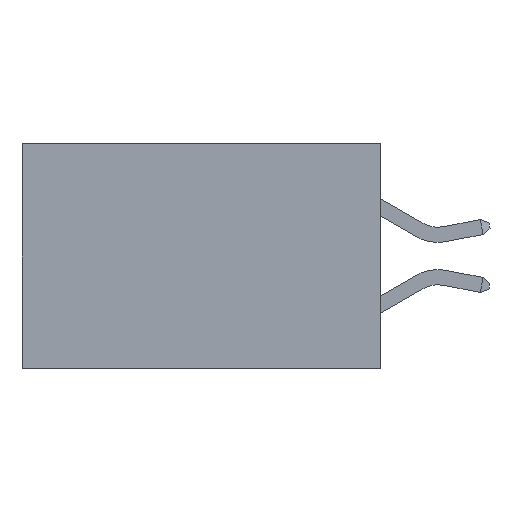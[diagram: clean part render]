
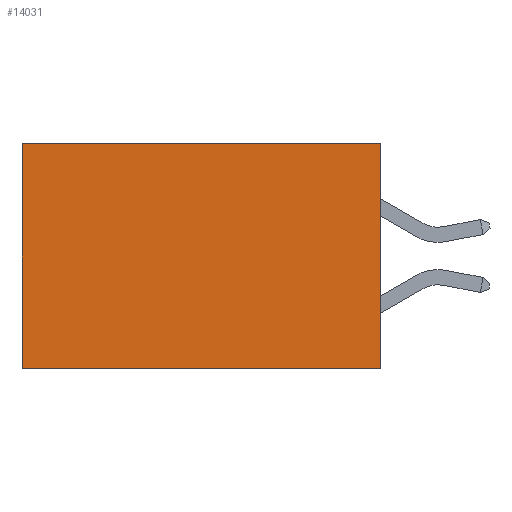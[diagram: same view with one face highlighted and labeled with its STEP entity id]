
A CAD part, left-side view. The second image highlights one B-rep face of the part: STEP entity #14031.
In plain terms, the highlighted planar face has unit normal (-1, 0, 0).
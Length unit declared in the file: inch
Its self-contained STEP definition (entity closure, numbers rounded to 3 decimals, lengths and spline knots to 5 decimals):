
#9 = EDGE_CURVE ( 'NONE', #14758, #8744, #9076, .T. ) ;
#296 = LINE ( 'NONE', #15651, #13128 ) ;
#1215 = AXIS2_PLACEMENT_3D ( 'NONE', #3953, #5200, #13872 ) ;
#1379 = VECTOR ( 'NONE', #11923, 39.37008 ) ;
#1619 = ORIENTED_EDGE ( 'NONE', *, *, #9367, .F. ) ;
#1762 = FACE_OUTER_BOUND ( 'NONE', #6398, .T. ) ;
#2040 = DIRECTION ( 'NONE',  ( 0., 1., 0. ) ) ;
#2311 = EDGE_CURVE ( 'NONE', #11370, #11696, #8771, .T. ) ;
#2517 = DIRECTION ( 'NONE',  ( 0., 0., -1. ) ) ;
#2707 = CARTESIAN_POINT ( 'NONE',  ( 0.277, 0., -0.37 ) ) ;
#3953 = CARTESIAN_POINT ( 'NONE',  ( 0.277, 0., -0.37 ) ) ;
#4618 = ORIENTED_EDGE ( 'NONE', *, *, #2311, .F. ) ;
#5199 = DIRECTION ( 'NONE',  ( 0., 1., 0. ) ) ;
#5200 = DIRECTION ( 'NONE',  ( 1., 0., 0. ) ) ;
#5404 = VECTOR ( 'NONE', #5199, 39.37008 ) ;
#6195 = EDGE_CURVE ( 'NONE', #11370, #14758, #296, .T. ) ;
#6398 = EDGE_LOOP ( 'NONE', ( #13866, #1619, #4618, #14774 ) ) ;
#6412 = PLANE ( 'NONE',  #1215 ) ;
#7197 = CARTESIAN_POINT ( 'NONE',  ( 0.277, 0., -0.37 ) ) ;
#8684 = LINE ( 'NONE', #2707, #5404 ) ;
#8744 = VERTEX_POINT ( 'NONE', #14230 ) ;
#8771 = LINE ( 'NONE', #12487, #1379 ) ;
#9076 = LINE ( 'NONE', #11350, #15661 ) ;
#9367 = EDGE_CURVE ( 'NONE', #11696, #8744, #8684, .T. ) ;
#11350 = CARTESIAN_POINT ( 'NONE',  ( 0.277, 0.59, -0.37 ) ) ;
#11370 = VERTEX_POINT ( 'NONE', #13971 ) ;
#11668 = CARTESIAN_POINT ( 'NONE',  ( 0.277, 0.59, 0. ) ) ;
#11696 = VERTEX_POINT ( 'NONE', #7197 ) ;
#11923 = DIRECTION ( 'NONE',  ( 0., 0., -1. ) ) ;
#12487 = CARTESIAN_POINT ( 'NONE',  ( 0.277, 0., -0.37 ) ) ;
#13128 = VECTOR ( 'NONE', #2040, 39.37008 ) ;
#13866 = ORIENTED_EDGE ( 'NONE', *, *, #9, .T. ) ;
#13872 = DIRECTION ( 'NONE',  ( 0., 0., -1. ) ) ;
#13971 = CARTESIAN_POINT ( 'NONE',  ( 0.277, 0., 0. ) ) ;
#14031 = ADVANCED_FACE ( 'NONE', ( #1762 ), #6412, .F. ) ;
#14230 = CARTESIAN_POINT ( 'NONE',  ( 0.277, 0.59, -0.37 ) ) ;
#14758 = VERTEX_POINT ( 'NONE', #11668 ) ;
#14774 = ORIENTED_EDGE ( 'NONE', *, *, #6195, .T. ) ;
#15651 = CARTESIAN_POINT ( 'NONE',  ( 0.277, 0., 0. ) ) ;
#15661 = VECTOR ( 'NONE', #2517, 39.37008 ) ;
